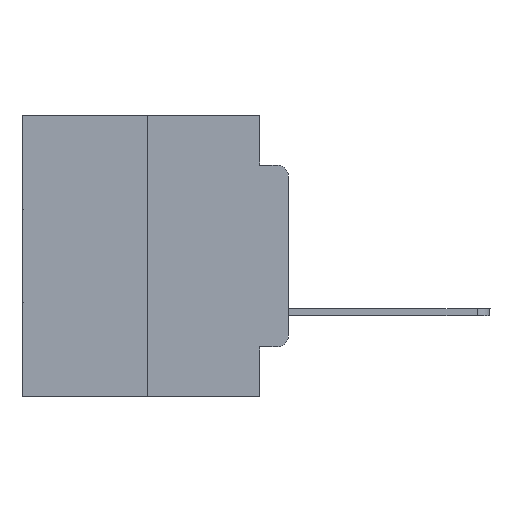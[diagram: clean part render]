
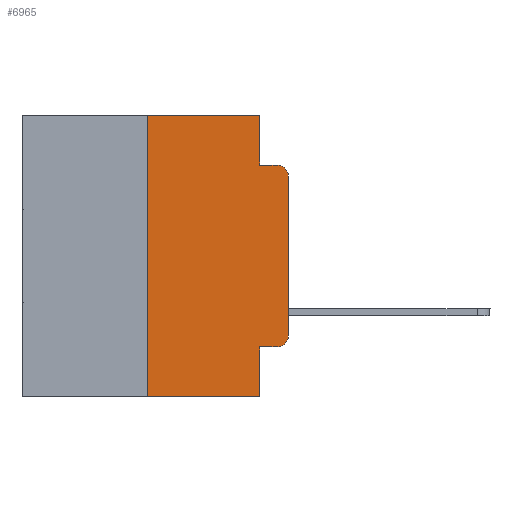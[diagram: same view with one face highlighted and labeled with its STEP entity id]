
A CAD part, left-side view. The second image highlights one B-rep face of the part: STEP entity #6965.
In plain terms, the highlighted planar face has unit normal (-1, 0, 0).
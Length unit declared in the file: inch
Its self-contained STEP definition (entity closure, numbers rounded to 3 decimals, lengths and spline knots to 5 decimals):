
#72 = VECTOR ( 'NONE', #19144, 39.37008 ) ;
#483 = CARTESIAN_POINT ( 'NONE',  ( 0., 0., -0.3915 ) ) ;
#936 = DIRECTION ( 'NONE',  ( 0., 0., 1. ) ) ;
#1201 = ORIENTED_EDGE ( 'NONE', *, *, #21601, .T. ) ;
#1284 = LINE ( 'NONE', #25970, #3765 ) ;
#1987 = CARTESIAN_POINT ( 'NONE',  ( 0., 0.02, -0.4115 ) ) ;
#2422 = CARTESIAN_POINT ( 'NONE',  ( 0., 0.051, -0.4115 ) ) ;
#2843 = CARTESIAN_POINT ( 'NONE',  ( 0., 0.02, -0.3915 ) ) ;
#3187 = EDGE_CURVE ( 'NONE', #27307, #7572, #12209, .T. ) ;
#3374 = DIRECTION ( 'NONE',  ( 0., 0., 1. ) ) ;
#3765 = VECTOR ( 'NONE', #3374, 39.37008 ) ;
#3910 = ORIENTED_EDGE ( 'NONE', *, *, #20132, .F. ) ;
#4082 = CARTESIAN_POINT ( 'NONE',  ( 0., 0.051, -0.4115 ) ) ;
#4780 = CARTESIAN_POINT ( 'NONE',  ( 0., 0.051, -0.0885 ) ) ;
#4805 = DIRECTION ( 'NONE',  ( -1., 0., 0. ) ) ;
#5293 = EDGE_CURVE ( 'NONE', #23804, #11421, #8300, .T. ) ;
#5670 = EDGE_CURVE ( 'NONE', #16270, #7572, #21637, .T. ) ;
#5776 = VECTOR ( 'NONE', #13799, 39.37008 ) ;
#6197 = CARTESIAN_POINT ( 'NONE',  ( 0., 0.473, 0. ) ) ;
#6715 = VERTEX_POINT ( 'NONE', #17806 ) ;
#6787 = CIRCLE ( 'NONE', #11150, 0.02 ) ;
#6965 = ADVANCED_FACE ( 'NONE', ( #20129 ), #16824, .F. ) ;
#7067 = CARTESIAN_POINT ( 'NONE',  ( 0., 0., -0.1085 ) ) ;
#7572 = VERTEX_POINT ( 'NONE', #26130 ) ;
#8300 = LINE ( 'NONE', #24653, #27640 ) ;
#8358 = EDGE_CURVE ( 'NONE', #6715, #11421, #10587, .T. ) ;
#9063 = VECTOR ( 'NONE', #11025, 39.37008 ) ;
#9477 = DIRECTION ( 'NONE',  ( 0., -1., 0. ) ) ;
#10029 = CARTESIAN_POINT ( 'NONE',  ( 0., 0.25, 0. ) ) ;
#10587 = LINE ( 'NONE', #14569, #72 ) ;
#10660 = ORIENTED_EDGE ( 'NONE', *, *, #5670, .T. ) ;
#10758 = VECTOR ( 'NONE', #936, 39.37008 ) ;
#11025 = DIRECTION ( 'NONE',  ( 0., 0., -1. ) ) ;
#11150 = AXIS2_PLACEMENT_3D ( 'NONE', #2843, #4805, #20509 ) ;
#11421 = VERTEX_POINT ( 'NONE', #20105 ) ;
#12209 = LINE ( 'NONE', #18376, #15744 ) ;
#12979 = ORIENTED_EDGE ( 'NONE', *, *, #3187, .F. ) ;
#13432 = AXIS2_PLACEMENT_3D ( 'NONE', #19392, #19204, #28487 ) ;
#13637 = AXIS2_PLACEMENT_3D ( 'NONE', #6197, #28771, #27025 ) ;
#13791 = DIRECTION ( 'NONE',  ( 0., -1., 0. ) ) ;
#13799 = DIRECTION ( 'NONE',  ( 0., -1., 0. ) ) ;
#14074 = EDGE_CURVE ( 'NONE', #6715, #22228, #16732, .T. ) ;
#14366 = EDGE_LOOP ( 'NONE', ( #1201, #10660, #12979, #3910, #21450, #14422, #27922, #15885, #15298, #18954 ) ) ;
#14388 = CARTESIAN_POINT ( 'NONE',  ( 0., 0.25, 0. ) ) ;
#14422 = ORIENTED_EDGE ( 'NONE', *, *, #14074, .F. ) ;
#14569 = CARTESIAN_POINT ( 'NONE',  ( 0., 0.473, -0.5 ) ) ;
#15045 = EDGE_CURVE ( 'NONE', #21862, #23391, #6787, .T. ) ;
#15298 = ORIENTED_EDGE ( 'NONE', *, *, #29076, .T. ) ;
#15744 = VECTOR ( 'NONE', #9477, 39.37008 ) ;
#15885 = ORIENTED_EDGE ( 'NONE', *, *, #5293, .F. ) ;
#16270 = VERTEX_POINT ( 'NONE', #7067 ) ;
#16732 = LINE ( 'NONE', #14388, #10758 ) ;
#16824 = PLANE ( 'NONE',  #13637 ) ;
#17735 = LINE ( 'NONE', #2422, #5776 ) ;
#17806 = CARTESIAN_POINT ( 'NONE',  ( 0., 0.25, -0.5 ) ) ;
#18376 = CARTESIAN_POINT ( 'NONE',  ( 0., 0.051, -0.0885 ) ) ;
#18473 = CARTESIAN_POINT ( 'NONE',  ( 0., 0.473, 0. ) ) ;
#18954 = ORIENTED_EDGE ( 'NONE', *, *, #15045, .T. ) ;
#19144 = DIRECTION ( 'NONE',  ( 0., -1., 0. ) ) ;
#19204 = DIRECTION ( 'NONE',  ( -1., 0., 0. ) ) ;
#19392 = CARTESIAN_POINT ( 'NONE',  ( 0., 0.02, -0.1085 ) ) ;
#19562 = LINE ( 'NONE', #22395, #9063 ) ;
#19630 = VECTOR ( 'NONE', #13791, 39.37008 ) ;
#20105 = CARTESIAN_POINT ( 'NONE',  ( 0., 0.051, -0.5 ) ) ;
#20129 = FACE_OUTER_BOUND ( 'NONE', #14366, .T. ) ;
#20132 = EDGE_CURVE ( 'NONE', #27691, #27307, #19562, .T. ) ;
#20509 = DIRECTION ( 'NONE',  ( 0., 0., -1. ) ) ;
#20684 = LINE ( 'NONE', #18473, #19630 ) ;
#21450 = ORIENTED_EDGE ( 'NONE', *, *, #26120, .F. ) ;
#21601 = EDGE_CURVE ( 'NONE', #23391, #16270, #1284, .T. ) ;
#21637 = CIRCLE ( 'NONE', #13432, 0.02 ) ;
#21862 = VERTEX_POINT ( 'NONE', #1987 ) ;
#21864 = CARTESIAN_POINT ( 'NONE',  ( 0., 0.051, 0. ) ) ;
#22228 = VERTEX_POINT ( 'NONE', #10029 ) ;
#22395 = CARTESIAN_POINT ( 'NONE',  ( 0., 0.051, 0. ) ) ;
#23391 = VERTEX_POINT ( 'NONE', #483 ) ;
#23804 = VERTEX_POINT ( 'NONE', #4082 ) ;
#24456 = DIRECTION ( 'NONE',  ( 0., 0., -1. ) ) ;
#24653 = CARTESIAN_POINT ( 'NONE',  ( 0., 0.051, 0. ) ) ;
#25970 = CARTESIAN_POINT ( 'NONE',  ( 0., 0., 0. ) ) ;
#26120 = EDGE_CURVE ( 'NONE', #22228, #27691, #20684, .T. ) ;
#26130 = CARTESIAN_POINT ( 'NONE',  ( 0., 0.02, -0.0885 ) ) ;
#27025 = DIRECTION ( 'NONE',  ( 0., 0., -1. ) ) ;
#27307 = VERTEX_POINT ( 'NONE', #4780 ) ;
#27640 = VECTOR ( 'NONE', #24456, 39.37008 ) ;
#27691 = VERTEX_POINT ( 'NONE', #21864 ) ;
#27922 = ORIENTED_EDGE ( 'NONE', *, *, #8358, .T. ) ;
#28487 = DIRECTION ( 'NONE',  ( 0., 0., -1. ) ) ;
#28771 = DIRECTION ( 'NONE',  ( 1., 0., 0. ) ) ;
#29076 = EDGE_CURVE ( 'NONE', #23804, #21862, #17735, .T. ) ;
